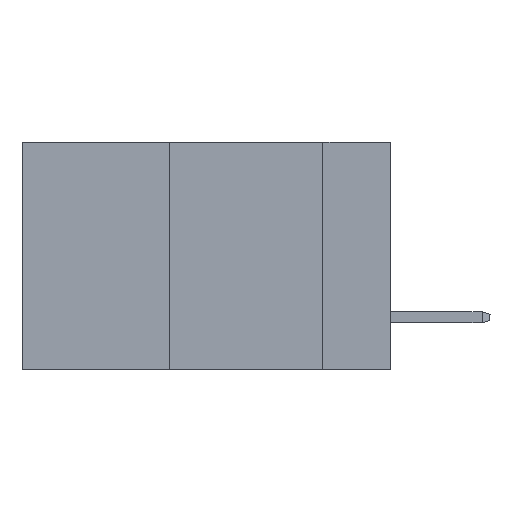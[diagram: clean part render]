
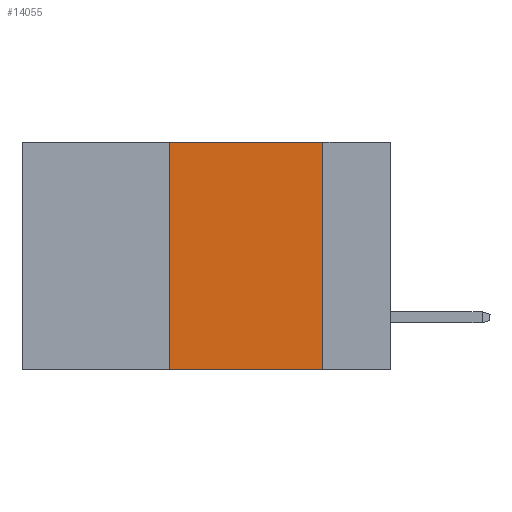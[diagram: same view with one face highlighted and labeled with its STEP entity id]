
A CAD part, left-side view. The second image highlights one B-rep face of the part: STEP entity #14055.
In plain terms, the highlighted planar face has unit normal (-1, 0, 0).
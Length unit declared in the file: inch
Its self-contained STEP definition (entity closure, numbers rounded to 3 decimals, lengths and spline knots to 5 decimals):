
#166 = CARTESIAN_POINT ( 'NONE',  ( 0., 0.6, 0. ) ) ;
#469 = EDGE_CURVE ( 'NONE', #9891, #1977, #22932, .T. ) ;
#729 = CARTESIAN_POINT ( 'NONE',  ( 0., 0.11, 0. ) ) ;
#1977 = VERTEX_POINT ( 'NONE', #4601 ) ;
#2140 = DIRECTION ( 'NONE',  ( 0., -1., 0. ) ) ;
#2233 = EDGE_LOOP ( 'NONE', ( #18964, #13979, #17899, #16030 ) ) ;
#3201 = AXIS2_PLACEMENT_3D ( 'NONE', #166, #3929, #12691 ) ;
#3518 = LINE ( 'NONE', #19949, #10521 ) ;
#3929 = DIRECTION ( 'NONE',  ( 1., 0., 0. ) ) ;
#4209 = FACE_OUTER_BOUND ( 'NONE', #2233, .T. ) ;
#4601 = CARTESIAN_POINT ( 'NONE',  ( 0., 0.36, 0. ) ) ;
#5848 = EDGE_CURVE ( 'NONE', #1977, #15812, #3518, .T. ) ;
#8365 = VECTOR ( 'NONE', #18524, 39.37008 ) ;
#8424 = EDGE_CURVE ( 'NONE', #9891, #17713, #9250, .T. ) ;
#8702 = VECTOR ( 'NONE', #11910, 39.37008 ) ;
#8977 = CARTESIAN_POINT ( 'NONE',  ( 0., 0.36, 0. ) ) ;
#9250 = LINE ( 'NONE', #20693, #8702 ) ;
#9891 = VERTEX_POINT ( 'NONE', #14191 ) ;
#10521 = VECTOR ( 'NONE', #2140, 39.37008 ) ;
#10591 = PLANE ( 'NONE',  #3201 ) ;
#11092 = EDGE_CURVE ( 'NONE', #15812, #17713, #12503, .T. ) ;
#11910 = DIRECTION ( 'NONE',  ( 0., -1., 0. ) ) ;
#12503 = LINE ( 'NONE', #22959, #17245 ) ;
#12691 = DIRECTION ( 'NONE',  ( 0., 0., -1. ) ) ;
#13979 = ORIENTED_EDGE ( 'NONE', *, *, #5848, .F. ) ;
#14055 = ADVANCED_FACE ( 'NONE', ( #4209 ), #10591, .F. ) ;
#14191 = CARTESIAN_POINT ( 'NONE',  ( 0., 0.36, -0.37 ) ) ;
#15812 = VERTEX_POINT ( 'NONE', #729 ) ;
#16030 = ORIENTED_EDGE ( 'NONE', *, *, #8424, .T. ) ;
#17245 = VECTOR ( 'NONE', #20909, 39.37008 ) ;
#17506 = CARTESIAN_POINT ( 'NONE',  ( 0., 0.11, -0.37 ) ) ;
#17713 = VERTEX_POINT ( 'NONE', #17506 ) ;
#17899 = ORIENTED_EDGE ( 'NONE', *, *, #469, .F. ) ;
#18524 = DIRECTION ( 'NONE',  ( 0., 0., 1. ) ) ;
#18964 = ORIENTED_EDGE ( 'NONE', *, *, #11092, .F. ) ;
#19949 = CARTESIAN_POINT ( 'NONE',  ( 0., 0.6, 0. ) ) ;
#20693 = CARTESIAN_POINT ( 'NONE',  ( 0., 0.6, -0.37 ) ) ;
#20909 = DIRECTION ( 'NONE',  ( 0., 0., -1. ) ) ;
#22932 = LINE ( 'NONE', #8977, #8365 ) ;
#22959 = CARTESIAN_POINT ( 'NONE',  ( 0., 0.11, 0. ) ) ;
